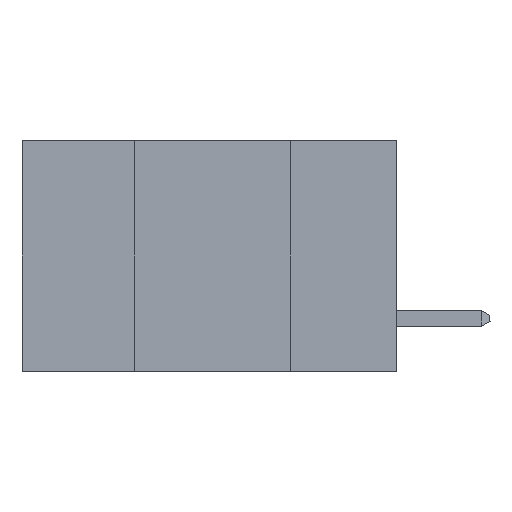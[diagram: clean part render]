
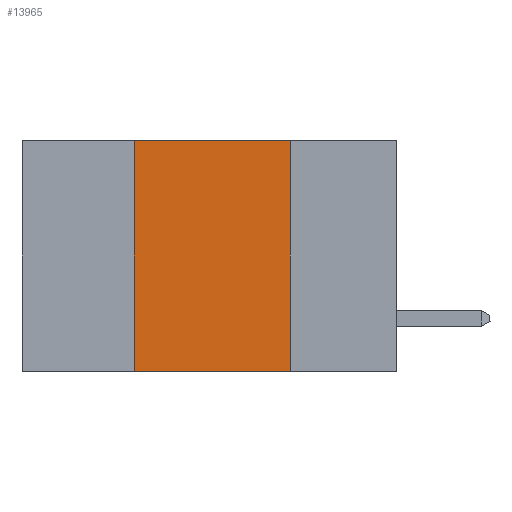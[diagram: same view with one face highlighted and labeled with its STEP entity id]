
A CAD part, left-side view. The second image highlights one B-rep face of the part: STEP entity #13965.
In plain terms, the highlighted planar face has unit normal (-1, 0, 0).
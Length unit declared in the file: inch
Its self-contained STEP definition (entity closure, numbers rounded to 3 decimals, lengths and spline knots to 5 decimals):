
#140 = CARTESIAN_POINT ( 'NONE',  ( 0., 0.6, -0.37 ) ) ;
#231 = DIRECTION ( 'NONE',  ( 0., -1., 0. ) ) ;
#1362 = CARTESIAN_POINT ( 'NONE',  ( 0., 0.17, -0.37 ) ) ;
#1890 = EDGE_CURVE ( 'NONE', #5868, #18990, #21801, .T. ) ;
#3569 = ORIENTED_EDGE ( 'NONE', *, *, #19396, .F. ) ;
#3824 = EDGE_LOOP ( 'NONE', ( #20790, #3569, #5570, #10857 ) ) ;
#5354 = DIRECTION ( 'NONE',  ( 0., 0., -1. ) ) ;
#5570 = ORIENTED_EDGE ( 'NONE', *, *, #1890, .F. ) ;
#5762 = DIRECTION ( 'NONE',  ( 0., 0., -1. ) ) ;
#5868 = VERTEX_POINT ( 'NONE', #18894 ) ;
#5928 = VERTEX_POINT ( 'NONE', #1362 ) ;
#8795 = VECTOR ( 'NONE', #5354, 39.37008 ) ;
#8918 = EDGE_CURVE ( 'NONE', #5868, #5928, #24044, .T. ) ;
#9461 = VERTEX_POINT ( 'NONE', #21231 ) ;
#9853 = DIRECTION ( 'NONE',  ( 0., -1., 0. ) ) ;
#10857 = ORIENTED_EDGE ( 'NONE', *, *, #8918, .T. ) ;
#11613 = VECTOR ( 'NONE', #9853, 39.37008 ) ;
#12249 = LINE ( 'NONE', #25158, #11613 ) ;
#13509 = PLANE ( 'NONE',  #16916 ) ;
#13775 = VECTOR ( 'NONE', #231, 39.37008 ) ;
#13965 = ADVANCED_FACE ( 'NONE', ( #20096 ), #13509, .F. ) ;
#14605 = CARTESIAN_POINT ( 'NONE',  ( 0., 0.42, 0. ) ) ;
#15422 = CARTESIAN_POINT ( 'NONE',  ( 0., 0.6, 0. ) ) ;
#15712 = EDGE_CURVE ( 'NONE', #9461, #5928, #24230, .T. ) ;
#16046 = VECTOR ( 'NONE', #19294, 39.37008 ) ;
#16916 = AXIS2_PLACEMENT_3D ( 'NONE', #15422, #17362, #5762 ) ;
#17362 = DIRECTION ( 'NONE',  ( 1., 0., 0. ) ) ;
#18894 = CARTESIAN_POINT ( 'NONE',  ( 0., 0.42, -0.37 ) ) ;
#18990 = VERTEX_POINT ( 'NONE', #14605 ) ;
#19294 = DIRECTION ( 'NONE',  ( 0., 0., 1. ) ) ;
#19396 = EDGE_CURVE ( 'NONE', #18990, #9461, #12249, .T. ) ;
#20096 = FACE_OUTER_BOUND ( 'NONE', #3824, .T. ) ;
#20790 = ORIENTED_EDGE ( 'NONE', *, *, #15712, .F. ) ;
#20842 = CARTESIAN_POINT ( 'NONE',  ( 0., 0.17, 0. ) ) ;
#21231 = CARTESIAN_POINT ( 'NONE',  ( 0., 0.17, 0. ) ) ;
#21303 = CARTESIAN_POINT ( 'NONE',  ( 0., 0.42, 0. ) ) ;
#21801 = LINE ( 'NONE', #21303, #16046 ) ;
#24044 = LINE ( 'NONE', #140, #13775 ) ;
#24230 = LINE ( 'NONE', #20842, #8795 ) ;
#25158 = CARTESIAN_POINT ( 'NONE',  ( 0., 0.6, 0. ) ) ;
